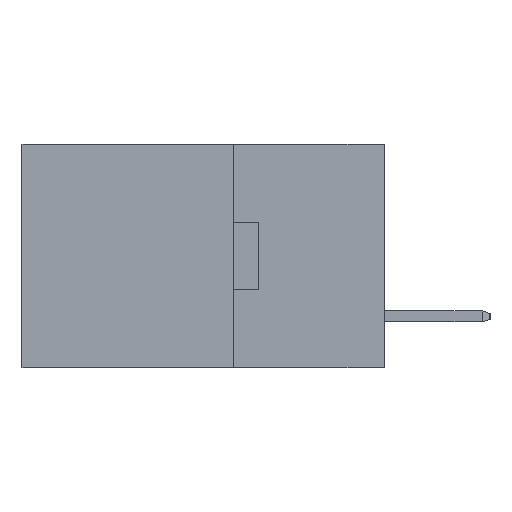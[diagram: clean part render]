
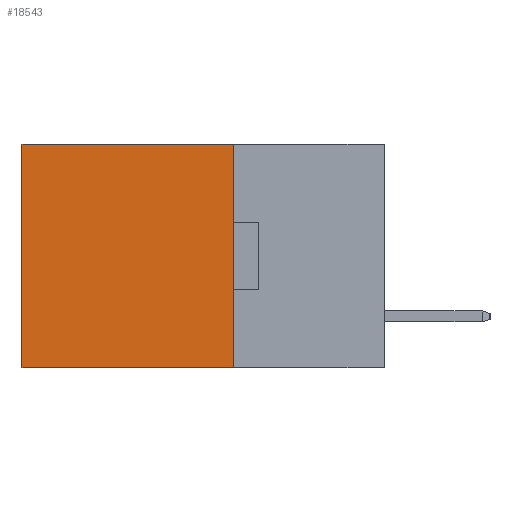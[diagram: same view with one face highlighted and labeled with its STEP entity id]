
A CAD part, left-side view. The second image highlights one B-rep face of the part: STEP entity #18543.
In plain terms, the highlighted planar face has unit normal (-1, 0, 0).
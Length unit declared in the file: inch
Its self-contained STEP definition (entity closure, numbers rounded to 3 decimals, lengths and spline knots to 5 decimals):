
#42 = LINE ( 'NONE', #18457, #21969 ) ;
#159 = EDGE_CURVE ( 'NONE', #15317, #346, #6585, .T. ) ;
#346 = VERTEX_POINT ( 'NONE', #12783 ) ;
#1409 = DIRECTION ( 'NONE',  ( 0., 1., 0. ) ) ;
#1508 = LINE ( 'NONE', #6797, #12936 ) ;
#3876 = EDGE_CURVE ( 'NONE', #6794, #11978, #1508, .T. ) ;
#4943 = CARTESIAN_POINT ( 'NONE',  ( 0.2615, 0.25, -0.37 ) ) ;
#5250 = ORIENTED_EDGE ( 'NONE', *, *, #3876, .F. ) ;
#6239 = CARTESIAN_POINT ( 'NONE',  ( 0.2615, 0.6, 0. ) ) ;
#6585 = LINE ( 'NONE', #27044, #12281 ) ;
#6794 = VERTEX_POINT ( 'NONE', #21887 ) ;
#6797 = CARTESIAN_POINT ( 'NONE',  ( 0.2615, 0.25, -0.37 ) ) ;
#7125 = DIRECTION ( 'NONE',  ( 1., 0., 0. ) ) ;
#7822 = ORIENTED_EDGE ( 'NONE', *, *, #25421, .F. ) ;
#11978 = VERTEX_POINT ( 'NONE', #19958 ) ;
#12281 = VECTOR ( 'NONE', #26951, 39.37008 ) ;
#12783 = CARTESIAN_POINT ( 'NONE',  ( 0.2615, 0.6, -0.37 ) ) ;
#12936 = VECTOR ( 'NONE', #17419, 39.37008 ) ;
#13089 = EDGE_CURVE ( 'NONE', #6794, #15317, #14196, .T. ) ;
#14196 = LINE ( 'NONE', #25373, #24609 ) ;
#15154 = AXIS2_PLACEMENT_3D ( 'NONE', #4943, #7125, #21878 ) ;
#15317 = VERTEX_POINT ( 'NONE', #6239 ) ;
#17419 = DIRECTION ( 'NONE',  ( 0., 0., -1. ) ) ;
#17451 = ORIENTED_EDGE ( 'NONE', *, *, #159, .T. ) ;
#17713 = PLANE ( 'NONE',  #15154 ) ;
#18457 = CARTESIAN_POINT ( 'NONE',  ( 0.2615, 0.25, -0.37 ) ) ;
#18543 = ADVANCED_FACE ( 'NONE', ( #25789 ), #17713, .F. ) ;
#19958 = CARTESIAN_POINT ( 'NONE',  ( 0.2615, 0.25, -0.37 ) ) ;
#21195 = DIRECTION ( 'NONE',  ( 0., 1., 0. ) ) ;
#21298 = EDGE_LOOP ( 'NONE', ( #17451, #7822, #5250, #26999 ) ) ;
#21878 = DIRECTION ( 'NONE',  ( 0., 0., -1. ) ) ;
#21887 = CARTESIAN_POINT ( 'NONE',  ( 0.2615, 0.25, 0. ) ) ;
#21969 = VECTOR ( 'NONE', #1409, 39.37008 ) ;
#24609 = VECTOR ( 'NONE', #21195, 39.37008 ) ;
#25373 = CARTESIAN_POINT ( 'NONE',  ( 0.2615, 0.25, 0. ) ) ;
#25421 = EDGE_CURVE ( 'NONE', #11978, #346, #42, .T. ) ;
#25789 = FACE_OUTER_BOUND ( 'NONE', #21298, .T. ) ;
#26951 = DIRECTION ( 'NONE',  ( 0., 0., -1. ) ) ;
#26999 = ORIENTED_EDGE ( 'NONE', *, *, #13089, .T. ) ;
#27044 = CARTESIAN_POINT ( 'NONE',  ( 0.2615, 0.6, -0.37 ) ) ;
